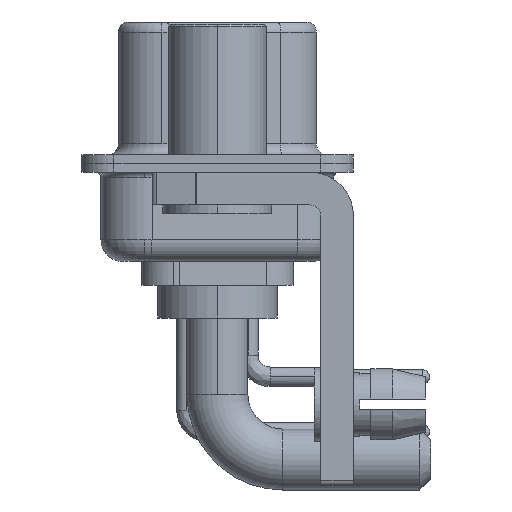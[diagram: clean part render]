
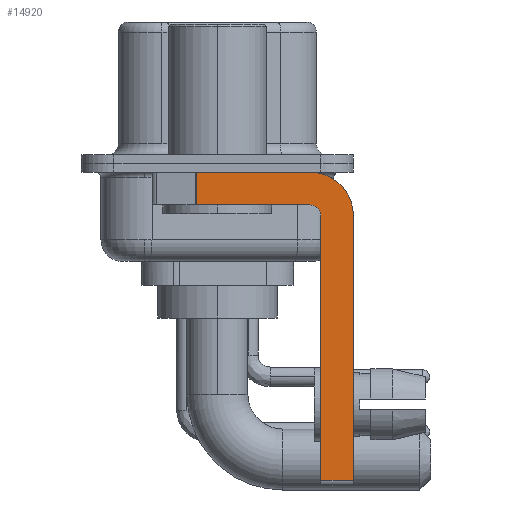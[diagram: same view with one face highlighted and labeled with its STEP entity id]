
A CAD part, left-side view. The second image highlights one B-rep face of the part: STEP entity #14920.
In plain terms, the highlighted planar face has unit normal (-1, 0, 0).
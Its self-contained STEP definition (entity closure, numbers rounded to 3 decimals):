
#418 = VECTOR ( 'NONE', #2185, 1000. ) ;
#1064 = EDGE_CURVE ( 'NONE', #26484, #22063, #22718, .T. ) ;
#1539 = ORIENTED_EDGE ( 'NONE', *, *, #10285, .F. ) ;
#1866 = ORIENTED_EDGE ( 'NONE', *, *, #1064, .F. ) ;
#2185 = DIRECTION ( 'NONE',  ( 0., 0., -1. ) ) ;
#2454 = CARTESIAN_POINT ( 'NONE',  ( -2.9, -6.25, -2.4 ) ) ;
#3861 = LINE ( 'NONE', #19857, #8630 ) ;
#4435 = CARTESIAN_POINT ( 'NONE',  ( -2.9, -4.75, -14.8 ) ) ;
#4556 = VECTOR ( 'NONE', #18542, 1000. ) ;
#4569 = EDGE_LOOP ( 'NONE', ( #13215, #25210, #22846, #25354, #1866, #23683, #8738, #1539 ) ) ;
#4932 = AXIS2_PLACEMENT_3D ( 'NONE', #17359, #11448, #21671 ) ;
#5165 = VERTEX_POINT ( 'NONE', #16930 ) ;
#5273 = LINE ( 'NONE', #21679, #24858 ) ;
#5739 = DIRECTION ( 'NONE',  ( 0., 0., -1. ) ) ;
#6137 = EDGE_CURVE ( 'NONE', #22063, #22701, #16934, .T. ) ;
#6405 = DIRECTION ( 'NONE',  ( 0., 0., -1. ) ) ;
#6864 = AXIS2_PLACEMENT_3D ( 'NONE', #22805, #14588, #6405 ) ;
#6979 = CARTESIAN_POINT ( 'NONE',  ( -2.9, -4.25, -14.55 ) ) ;
#8021 = DIRECTION ( 'NONE',  ( 1., 0., 0. ) ) ;
#8439 = CARTESIAN_POINT ( 'NONE',  ( -2.9, -6.25, -14.55 ) ) ;
#8630 = VECTOR ( 'NONE', #18097, 1000. ) ;
#8686 = PLANE ( 'NONE',  #6864 ) ;
#8738 = ORIENTED_EDGE ( 'NONE', *, *, #14356, .F. ) ;
#9387 = CARTESIAN_POINT ( 'NONE',  ( -2.9, -4.25, -0.4 ) ) ;
#9635 = CARTESIAN_POINT ( 'NONE',  ( -2.9, -4.25, -2.4 ) ) ;
#9791 = CARTESIAN_POINT ( 'NONE',  ( -2.9, 0.978, -1.9 ) ) ;
#9810 = VERTEX_POINT ( 'NONE', #9791 ) ;
#10235 = CARTESIAN_POINT ( 'NONE',  ( -2.9, -4.75, -14.55 ) ) ;
#10285 = EDGE_CURVE ( 'NONE', #14500, #5165, #13879, .T. ) ;
#10594 = VERTEX_POINT ( 'NONE', #15504 ) ;
#11448 = DIRECTION ( 'NONE',  ( -1., 0., 0. ) ) ;
#13215 = ORIENTED_EDGE ( 'NONE', *, *, #18664, .F. ) ;
#13530 = VERTEX_POINT ( 'NONE', #8439 ) ;
#13879 = CIRCLE ( 'NONE', #14305, 2. ) ;
#14270 = VECTOR ( 'NONE', #15424, 1000. ) ;
#14305 = AXIS2_PLACEMENT_3D ( 'NONE', #9635, #8021, #5739 ) ;
#14356 = EDGE_CURVE ( 'NONE', #5165, #13530, #20589, .T. ) ;
#14500 = VERTEX_POINT ( 'NONE', #9387 ) ;
#14588 = DIRECTION ( 'NONE',  ( 1., 0., 0. ) ) ;
#14920 = ADVANCED_FACE ( 'NONE', ( #16608 ), #8686, .F. ) ;
#15424 = DIRECTION ( 'NONE',  ( 0., -1., 0. ) ) ;
#15504 = CARTESIAN_POINT ( 'NONE',  ( -2.9, 0.978, -0.4 ) ) ;
#15590 = EDGE_CURVE ( 'NONE', #22701, #9810, #5273, .T. ) ;
#16608 = FACE_OUTER_BOUND ( 'NONE', #4569, .T. ) ;
#16930 = CARTESIAN_POINT ( 'NONE',  ( -2.9, -6.25, -2.4 ) ) ;
#16934 = CIRCLE ( 'NONE', #4932, 0.5 ) ;
#17359 = CARTESIAN_POINT ( 'NONE',  ( -2.9, -4.25, -2.4 ) ) ;
#17870 = CARTESIAN_POINT ( 'NONE',  ( -2.9, 3., -0.4 ) ) ;
#17975 = EDGE_CURVE ( 'NONE', #10594, #9810, #3861, .T. ) ;
#18097 = DIRECTION ( 'NONE',  ( 0., 0., -1. ) ) ;
#18542 = DIRECTION ( 'NONE',  ( 0., 0., 1. ) ) ;
#18664 = EDGE_CURVE ( 'NONE', #10594, #14500, #20025, .T. ) ;
#19104 = EDGE_CURVE ( 'NONE', #26484, #13530, #25408, .T. ) ;
#19643 = DIRECTION ( 'NONE',  ( 0., 1., 0. ) ) ;
#19672 = CARTESIAN_POINT ( 'NONE',  ( -2.9, -4.25, -1.9 ) ) ;
#19857 = CARTESIAN_POINT ( 'NONE',  ( -2.9, 0.978, -1.9 ) ) ;
#20025 = LINE ( 'NONE', #17870, #25433 ) ;
#20589 = LINE ( 'NONE', #2454, #418 ) ;
#21671 = DIRECTION ( 'NONE',  ( 0., 0., 1. ) ) ;
#21679 = CARTESIAN_POINT ( 'NONE',  ( -2.9, -4.25, -1.9 ) ) ;
#22063 = VERTEX_POINT ( 'NONE', #23893 ) ;
#22187 = DIRECTION ( 'NONE',  ( 0., -1., 0. ) ) ;
#22701 = VERTEX_POINT ( 'NONE', #19672 ) ;
#22718 = LINE ( 'NONE', #4435, #4556 ) ;
#22805 = CARTESIAN_POINT ( 'NONE',  ( -2.9, -4.25, -2.4 ) ) ;
#22846 = ORIENTED_EDGE ( 'NONE', *, *, #15590, .F. ) ;
#23683 = ORIENTED_EDGE ( 'NONE', *, *, #19104, .T. ) ;
#23893 = CARTESIAN_POINT ( 'NONE',  ( -2.9, -4.75, -2.4 ) ) ;
#24858 = VECTOR ( 'NONE', #19643, 1000. ) ;
#25210 = ORIENTED_EDGE ( 'NONE', *, *, #17975, .T. ) ;
#25354 = ORIENTED_EDGE ( 'NONE', *, *, #6137, .F. ) ;
#25408 = LINE ( 'NONE', #6979, #14270 ) ;
#25433 = VECTOR ( 'NONE', #22187, 1000. ) ;
#26484 = VERTEX_POINT ( 'NONE', #10235 ) ;
